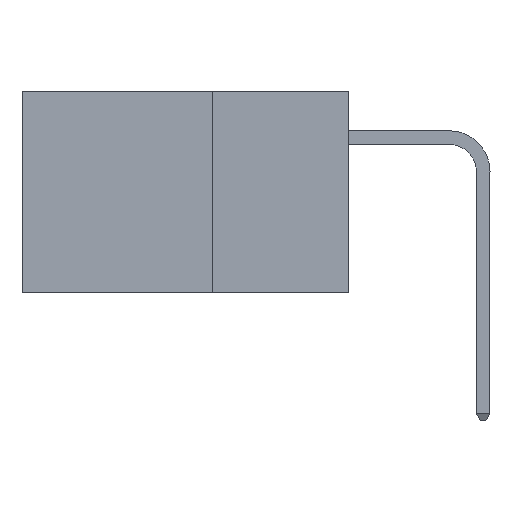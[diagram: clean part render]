
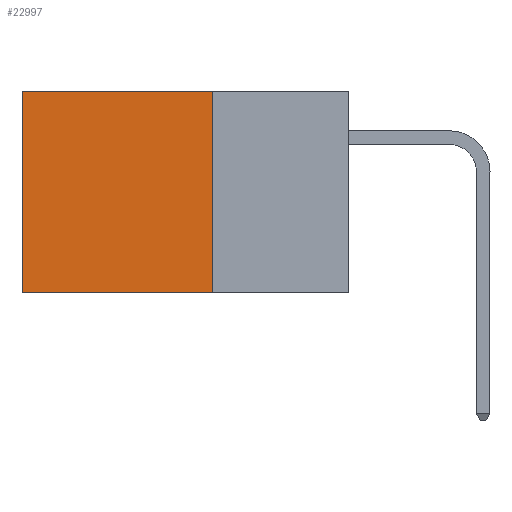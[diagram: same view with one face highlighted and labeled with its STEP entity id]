
A CAD part, left-side view. The second image highlights one B-rep face of the part: STEP entity #22997.
In plain terms, the highlighted planar face has unit normal (-1, 0, 0).
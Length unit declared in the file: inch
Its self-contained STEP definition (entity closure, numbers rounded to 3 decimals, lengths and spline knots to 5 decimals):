
#888 = LINE ( 'NONE', #26006, #25713 ) ;
#1426 = CARTESIAN_POINT ( 'NONE',  ( 0.2875, 0.25, -0.37 ) ) ;
#2323 = CARTESIAN_POINT ( 'NONE',  ( 0.2875, 0.25, -0.37 ) ) ;
#3076 = VECTOR ( 'NONE', #8347, 39.37008 ) ;
#4229 = VECTOR ( 'NONE', #16823, 39.37008 ) ;
#5479 = VERTEX_POINT ( 'NONE', #1426 ) ;
#6386 = EDGE_CURVE ( 'NONE', #5479, #17363, #21896, .T. ) ;
#6456 = EDGE_CURVE ( 'NONE', #19132, #5479, #11866, .T. ) ;
#6819 = CARTESIAN_POINT ( 'NONE',  ( 0.2875, 0.25, 0. ) ) ;
#8048 = CARTESIAN_POINT ( 'NONE',  ( 0.2875, 0.6, 0. ) ) ;
#8347 = DIRECTION ( 'NONE',  ( 0., 0., -1. ) ) ;
#9022 = ORIENTED_EDGE ( 'NONE', *, *, #19097, .T. ) ;
#9677 = DIRECTION ( 'NONE',  ( 0., 0., -1. ) ) ;
#11866 = LINE ( 'NONE', #30404, #4229 ) ;
#12351 = EDGE_LOOP ( 'NONE', ( #9022, #21669, #31870, #25817 ) ) ;
#13618 = VECTOR ( 'NONE', #35659, 39.37008 ) ;
#16823 = DIRECTION ( 'NONE',  ( 0., 0., -1. ) ) ;
#17363 = VERTEX_POINT ( 'NONE', #22560 ) ;
#18991 = LINE ( 'NONE', #33168, #3076 ) ;
#19097 = EDGE_CURVE ( 'NONE', #35428, #17363, #18991, .T. ) ;
#19132 = VERTEX_POINT ( 'NONE', #30664 ) ;
#20469 = DIRECTION ( 'NONE',  ( 0., 1., 0. ) ) ;
#21669 = ORIENTED_EDGE ( 'NONE', *, *, #6386, .F. ) ;
#21896 = LINE ( 'NONE', #2323, #13618 ) ;
#22560 = CARTESIAN_POINT ( 'NONE',  ( 0.2875, 0.6, -0.37 ) ) ;
#22997 = ADVANCED_FACE ( 'NONE', ( #34179 ), #23586, .F. ) ;
#23586 = PLANE ( 'NONE',  #27725 ) ;
#25713 = VECTOR ( 'NONE', #20469, 39.37008 ) ;
#25817 = ORIENTED_EDGE ( 'NONE', *, *, #32456, .T. ) ;
#26006 = CARTESIAN_POINT ( 'NONE',  ( 0.2875, 0.25, 0. ) ) ;
#26338 = DIRECTION ( 'NONE',  ( 1., 0., 0. ) ) ;
#27725 = AXIS2_PLACEMENT_3D ( 'NONE', #6819, #26338, #9677 ) ;
#30404 = CARTESIAN_POINT ( 'NONE',  ( 0.2875, 0.25, 0. ) ) ;
#30664 = CARTESIAN_POINT ( 'NONE',  ( 0.2875, 0.25, 0. ) ) ;
#31870 = ORIENTED_EDGE ( 'NONE', *, *, #6456, .F. ) ;
#32456 = EDGE_CURVE ( 'NONE', #19132, #35428, #888, .T. ) ;
#33168 = CARTESIAN_POINT ( 'NONE',  ( 0.2875, 0.6, 0. ) ) ;
#34179 = FACE_OUTER_BOUND ( 'NONE', #12351, .T. ) ;
#35428 = VERTEX_POINT ( 'NONE', #8048 ) ;
#35659 = DIRECTION ( 'NONE',  ( 0., 1., 0. ) ) ;
